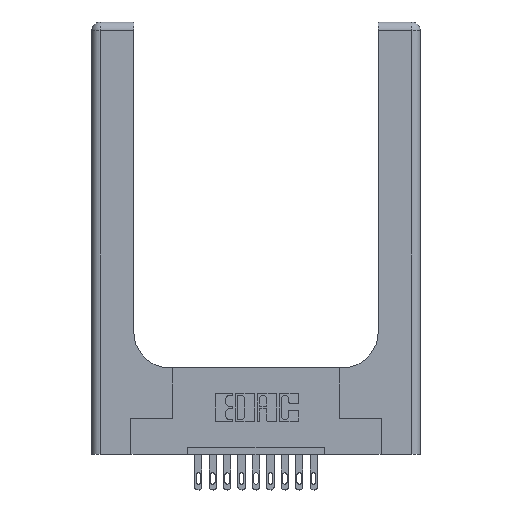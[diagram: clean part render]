
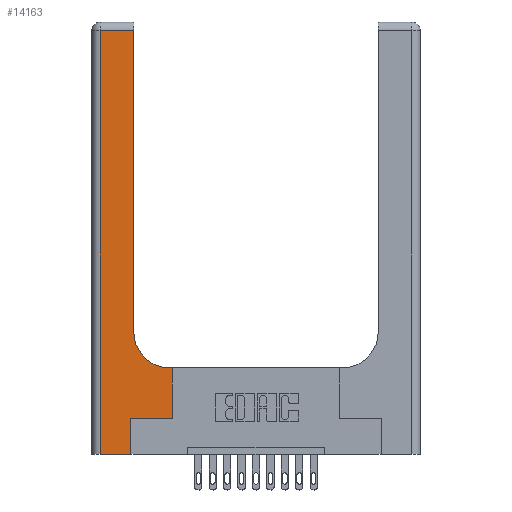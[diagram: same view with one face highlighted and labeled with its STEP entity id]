
A CAD part, top view. The second image highlights one B-rep face of the part: STEP entity #14163.
In plain terms, the highlighted planar face has unit normal (0, 0, 1).
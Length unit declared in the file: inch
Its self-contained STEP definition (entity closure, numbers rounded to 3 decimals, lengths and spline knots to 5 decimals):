
#165 = DIRECTION ( 'NONE',  ( 0., 0., -1. ) ) ;
#193 = CARTESIAN_POINT ( 'NONE',  ( 0.2915, 3., 0.37 ) ) ;
#205 = DIRECTION ( 'NONE',  ( 0., 0., -1. ) ) ;
#290 = VERTEX_POINT ( 'NONE', #14681 ) ;
#536 = CARTESIAN_POINT ( 'NONE',  ( 0.2915, 0.6, 0.37 ) ) ;
#888 = AXIS2_PLACEMENT_3D ( 'NONE', #4063, #165, #9045 ) ;
#1184 = VECTOR ( 'NONE', #6655, 39.37008 ) ;
#1190 = LINE ( 'NONE', #193, #12254 ) ;
#1289 = CARTESIAN_POINT ( 'NONE',  ( 0.2915, 0.85, 0.37 ) ) ;
#1392 = CARTESIAN_POINT ( 'NONE',  ( 0.5585, 0.25, 0.37 ) ) ;
#1626 = AXIS2_PLACEMENT_3D ( 'NONE', #9077, #205, #14129 ) ;
#2545 = CARTESIAN_POINT ( 'NONE',  ( 0.269, 0.25, 0.37 ) ) ;
#2790 = VECTOR ( 'NONE', #15624, 39.37008 ) ;
#2945 = LINE ( 'NONE', #9149, #1184 ) ;
#3814 = VERTEX_POINT ( 'NONE', #10373 ) ;
#3885 = LINE ( 'NONE', #15213, #15696 ) ;
#4019 = VECTOR ( 'NONE', #11088, 39.37008 ) ;
#4063 = CARTESIAN_POINT ( 'NONE',  ( 0.5415, 0.85, 0.37 ) ) ;
#4166 = DIRECTION ( 'NONE',  ( -1., 0., 0. ) ) ;
#4780 = EDGE_CURVE ( 'NONE', #12604, #14645, #3885, .T. ) ;
#5070 = FACE_OUTER_BOUND ( 'NONE', #8552, .T. ) ;
#5459 = ORIENTED_EDGE ( 'NONE', *, *, #4780, .T. ) ;
#5751 = CARTESIAN_POINT ( 'NONE',  ( 0., 2.94, 0.37 ) ) ;
#6477 = CIRCLE ( 'NONE', #888, 0.25 ) ;
#6655 = DIRECTION ( 'NONE',  ( 1., 0., 0. ) ) ;
#6747 = LINE ( 'NONE', #536, #11260 ) ;
#7237 = ORIENTED_EDGE ( 'NONE', *, *, #9886, .T. ) ;
#7329 = ORIENTED_EDGE ( 'NONE', *, *, #10408, .T. ) ;
#7426 = EDGE_CURVE ( 'NONE', #10292, #11670, #14993, .T. ) ;
#7431 = CARTESIAN_POINT ( 'NONE',  ( 0.269, 0., 0.37 ) ) ;
#7626 = CARTESIAN_POINT ( 'NONE',  ( 0.5585, 0.6, 0.37 ) ) ;
#7706 = DIRECTION ( 'NONE',  ( 0., 1., 0. ) ) ;
#8087 = EDGE_CURVE ( 'NONE', #13397, #8837, #1190, .T. ) ;
#8139 = LINE ( 'NONE', #14845, #4019 ) ;
#8552 = EDGE_LOOP ( 'NONE', ( #8756, #13721, #7237, #10255, #5459, #14512, #8791, #7329, #9966 ) ) ;
#8756 = ORIENTED_EDGE ( 'NONE', *, *, #8087, .T. ) ;
#8791 = ORIENTED_EDGE ( 'NONE', *, *, #7426, .T. ) ;
#8837 = VERTEX_POINT ( 'NONE', #15082 ) ;
#9002 = CARTESIAN_POINT ( 'NONE',  ( 0.06, 3., 0.37 ) ) ;
#9045 = DIRECTION ( 'NONE',  ( 1., 0., 0. ) ) ;
#9077 = CARTESIAN_POINT ( 'NONE',  ( 0., 3., 0.37 ) ) ;
#9149 = CARTESIAN_POINT ( 'NONE',  ( 0., 0., 0.37 ) ) ;
#9642 = VECTOR ( 'NONE', #12100, 39.37008 ) ;
#9886 = EDGE_CURVE ( 'NONE', #15791, #290, #15234, .T. ) ;
#9966 = ORIENTED_EDGE ( 'NONE', *, *, #13392, .T. ) ;
#10255 = ORIENTED_EDGE ( 'NONE', *, *, #11741, .T. ) ;
#10292 = VERTEX_POINT ( 'NONE', #1392 ) ;
#10373 = CARTESIAN_POINT ( 'NONE',  ( 0.5415, 0.6, 0.37 ) ) ;
#10408 = EDGE_CURVE ( 'NONE', #11670, #3814, #6747, .T. ) ;
#10822 = EDGE_CURVE ( 'NONE', #8837, #15791, #15960, .T. ) ;
#11088 = DIRECTION ( 'NONE',  ( 1., 0., 0. ) ) ;
#11260 = VECTOR ( 'NONE', #4166, 39.37008 ) ;
#11279 = VECTOR ( 'NONE', #14051, 39.37008 ) ;
#11670 = VERTEX_POINT ( 'NONE', #7626 ) ;
#11741 = EDGE_CURVE ( 'NONE', #290, #12604, #2945, .T. ) ;
#11953 = CARTESIAN_POINT ( 'NONE',  ( 0.5585, 0.25, 0.37 ) ) ;
#12100 = DIRECTION ( 'NONE',  ( -1., 0., 0. ) ) ;
#12254 = VECTOR ( 'NONE', #7706, 39.37008 ) ;
#12604 = VERTEX_POINT ( 'NONE', #7431 ) ;
#12980 = PLANE ( 'NONE',  #1626 ) ;
#13392 = EDGE_CURVE ( 'NONE', #3814, #13397, #6477, .T. ) ;
#13397 = VERTEX_POINT ( 'NONE', #1289 ) ;
#13721 = ORIENTED_EDGE ( 'NONE', *, *, #10822, .T. ) ;
#14051 = DIRECTION ( 'NONE',  ( 0., -1., 0. ) ) ;
#14069 = DIRECTION ( 'NONE',  ( 0., 1., 0. ) ) ;
#14129 = DIRECTION ( 'NONE',  ( -1., 0., 0. ) ) ;
#14163 = ADVANCED_FACE ( 'NONE', ( #5070 ), #12980, .F. ) ;
#14512 = ORIENTED_EDGE ( 'NONE', *, *, #15775, .T. ) ;
#14645 = VERTEX_POINT ( 'NONE', #2545 ) ;
#14681 = CARTESIAN_POINT ( 'NONE',  ( 0.06, 0., 0.37 ) ) ;
#14845 = CARTESIAN_POINT ( 'NONE',  ( 0.269, 0.25, 0.37 ) ) ;
#14993 = LINE ( 'NONE', #11953, #2790 ) ;
#15082 = CARTESIAN_POINT ( 'NONE',  ( 0.2915, 2.94, 0.37 ) ) ;
#15213 = CARTESIAN_POINT ( 'NONE',  ( 0.269, 0., 0.37 ) ) ;
#15234 = LINE ( 'NONE', #9002, #11279 ) ;
#15624 = DIRECTION ( 'NONE',  ( 0., 1., 0. ) ) ;
#15696 = VECTOR ( 'NONE', #14069, 39.37008 ) ;
#15775 = EDGE_CURVE ( 'NONE', #14645, #10292, #8139, .T. ) ;
#15791 = VERTEX_POINT ( 'NONE', #16306 ) ;
#15960 = LINE ( 'NONE', #5751, #9642 ) ;
#16306 = CARTESIAN_POINT ( 'NONE',  ( 0.06, 2.94, 0.37 ) ) ;
